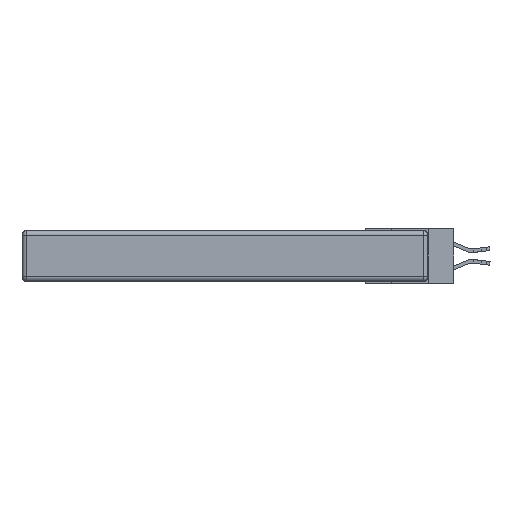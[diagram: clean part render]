
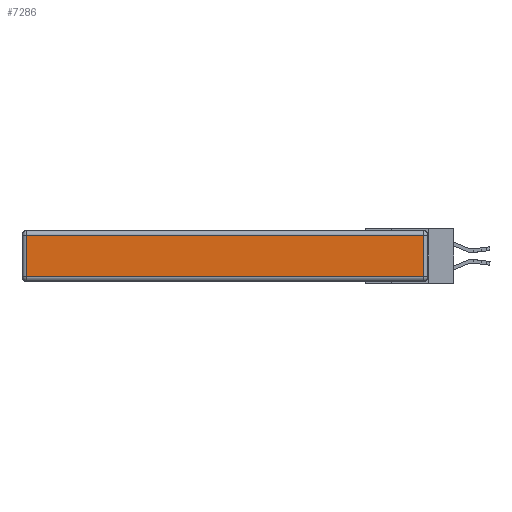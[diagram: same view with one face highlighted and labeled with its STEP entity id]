
A CAD part, left-side view. The second image highlights one B-rep face of the part: STEP entity #7286.
In plain terms, the highlighted planar face has unit normal (-1, 0, 0).
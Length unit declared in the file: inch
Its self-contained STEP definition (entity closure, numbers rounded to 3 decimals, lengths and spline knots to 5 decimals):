
#236 = CARTESIAN_POINT ( 'NONE',  ( 0., 2.72, -0.313 ) ) ;
#466 = VECTOR ( 'NONE', #12426, 39.37008 ) ;
#536 = EDGE_CURVE ( 'NONE', #3697, #17489, #2471, .T. ) ;
#2471 = LINE ( 'NONE', #28119, #10790 ) ;
#2918 = PLANE ( 'NONE',  #21199 ) ;
#3697 = VERTEX_POINT ( 'NONE', #23246 ) ;
#4711 = FACE_OUTER_BOUND ( 'NONE', #5873, .T. ) ;
#5873 = EDGE_LOOP ( 'NONE', ( #9483, #25051, #28477, #9674 ) ) ;
#7286 = ADVANCED_FACE ( 'NONE', ( #4711 ), #2918, .T. ) ;
#9483 = ORIENTED_EDGE ( 'NONE', *, *, #19926, .T. ) ;
#9674 = ORIENTED_EDGE ( 'NONE', *, *, #536, .T. ) ;
#10137 = DIRECTION ( 'NONE',  ( 0., 0., 1. ) ) ;
#10790 = VECTOR ( 'NONE', #12082, 39.37008 ) ;
#11005 = LINE ( 'NONE', #25209, #26994 ) ;
#11414 = DIRECTION ( 'NONE',  ( 0., -1., 0. ) ) ;
#11941 = LINE ( 'NONE', #24113, #26476 ) ;
#12082 = DIRECTION ( 'NONE',  ( 0., 0., -1. ) ) ;
#12416 = EDGE_CURVE ( 'NONE', #18320, #3697, #27278, .T. ) ;
#12426 = DIRECTION ( 'NONE',  ( 0., 1., 0. ) ) ;
#14652 = VERTEX_POINT ( 'NONE', #18772 ) ;
#17489 = VERTEX_POINT ( 'NONE', #236 ) ;
#18320 = VERTEX_POINT ( 'NONE', #29908 ) ;
#18772 = CARTESIAN_POINT ( 'NONE',  ( 0., 0.03, -0.313 ) ) ;
#19926 = EDGE_CURVE ( 'NONE', #17489, #14652, #11005, .T. ) ;
#21199 = AXIS2_PLACEMENT_3D ( 'NONE', #28642, #23859, #26212 ) ;
#23246 = CARTESIAN_POINT ( 'NONE',  ( 0., 2.72, -0.03 ) ) ;
#23859 = DIRECTION ( 'NONE',  ( -1., 0., 0. ) ) ;
#24113 = CARTESIAN_POINT ( 'NONE',  ( 0., 0.03, -0.343 ) ) ;
#25051 = ORIENTED_EDGE ( 'NONE', *, *, #26600, .T. ) ;
#25209 = CARTESIAN_POINT ( 'NONE',  ( 0., 0., -0.313 ) ) ;
#26212 = DIRECTION ( 'NONE',  ( 0., 0., 1. ) ) ;
#26307 = CARTESIAN_POINT ( 'NONE',  ( 0., 2.75, -0.03 ) ) ;
#26476 = VECTOR ( 'NONE', #10137, 39.37008 ) ;
#26600 = EDGE_CURVE ( 'NONE', #14652, #18320, #11941, .T. ) ;
#26994 = VECTOR ( 'NONE', #11414, 39.37008 ) ;
#27278 = LINE ( 'NONE', #26307, #466 ) ;
#28119 = CARTESIAN_POINT ( 'NONE',  ( 0., 2.72, -0.343 ) ) ;
#28477 = ORIENTED_EDGE ( 'NONE', *, *, #12416, .T. ) ;
#28642 = CARTESIAN_POINT ( 'NONE',  ( 0., 0., -0.343 ) ) ;
#29908 = CARTESIAN_POINT ( 'NONE',  ( 0., 0.03, -0.03 ) ) ;
